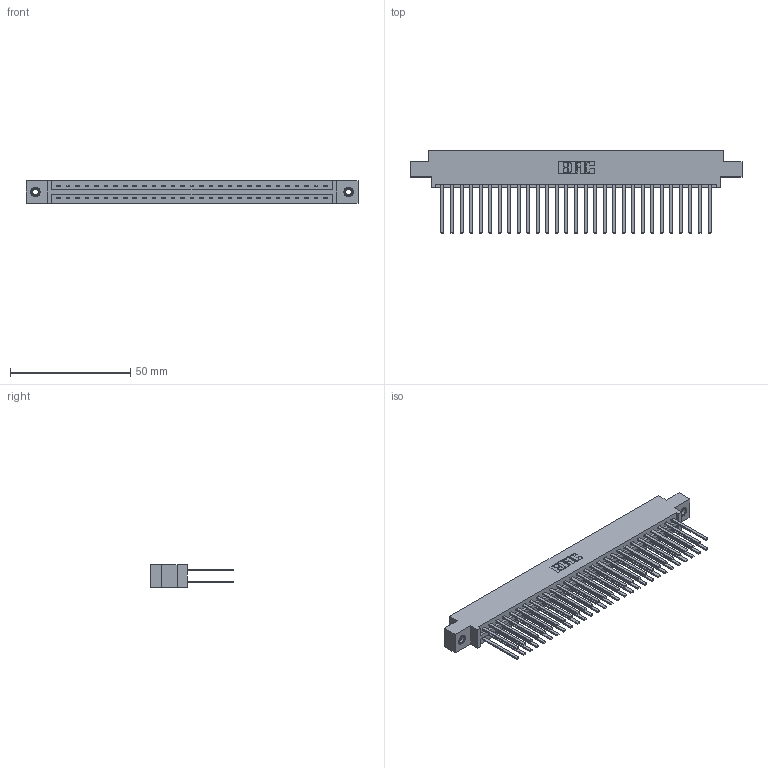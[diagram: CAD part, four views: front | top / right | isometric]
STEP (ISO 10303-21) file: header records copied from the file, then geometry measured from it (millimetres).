
FILE_DESCRIPTION (( 'STEP AP203' ), '1' );
FILE_NAME ('387-058-544-807.STEP', '2018-09-21T01:51:21', ( '' ), ( '' ), 'SwSTEP 2.0', 'SolidWorks 2016', '' );
FILE_SCHEMA (( 'CONFIG_CONTROL_DESIGN' ));
Length unit declared in the file: inch
Products named in the file (4): 337 Part_0.170 Offset - 0.156 Dia-TI; 345-292-001_345-293-144; 345-250-001_345-250-005-103; 387-058-544-807
Assembly tree (61 placements, depth 2):
  387-058-544-807
    337 Part_0.170 Offset - 0.156 Dia-TI
    345-292-001_345-293-144  x58
    345-250-001_345-250-005-103  x2
Bounding box: 137.92 x 34.3 x 9.4 mm (x, y, z)
Volume: 15044.3 mm3; surface area: 19681.1 mm2
Topology: 61 solids, 61 shells, 2962 faces, 8753 edges, 5750 vertices
Faces by surface type: plane 2078, cylinder 868, cone 12, torus 4
Entity records: 25300 total; most frequent: CARTESIAN_POINT 4253, ORIENTED_EDGE 4182, DIRECTION 3669, EDGE_CURVE 2091, VECTOR 1947, LINE 1947, VERTEX_POINT 1388, AXIS2_PLACEMENT_3D 861
